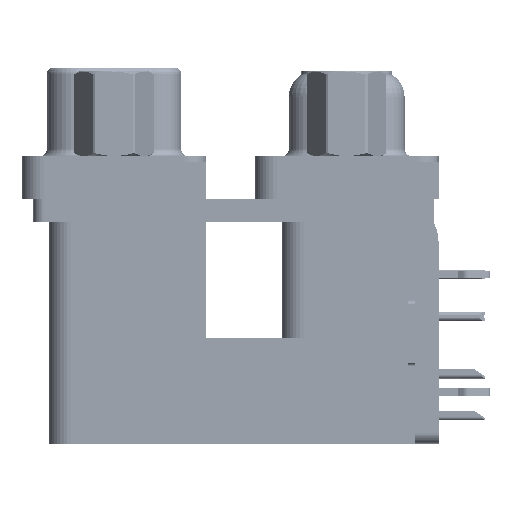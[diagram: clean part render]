
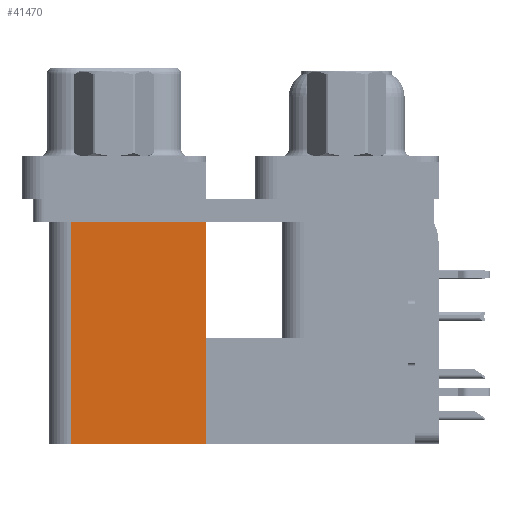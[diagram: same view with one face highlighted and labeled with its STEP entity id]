
A CAD part, left-side view. The second image highlights one B-rep face of the part: STEP entity #41470.
In plain terms, the highlighted planar face has unit normal (-1, 0, 0).
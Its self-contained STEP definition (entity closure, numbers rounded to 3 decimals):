
#2677 = EDGE_CURVE ( 'NONE', #49202, #59503, #44409, .T. ) ;
#3089 = EDGE_CURVE ( 'NONE', #24896, #7739, #49292, .T. ) ;
#5313 = CARTESIAN_POINT ( 'NONE',  ( 3.7, 9.6, -2.5 ) ) ;
#6377 = DIRECTION ( 'NONE',  ( 0., 0., -1. ) ) ;
#7739 = VERTEX_POINT ( 'NONE', #27088 ) ;
#9005 = LINE ( 'NONE', #17838, #18679 ) ;
#10030 = EDGE_LOOP ( 'NONE', ( #37730, #56517, #49188, #27973 ) ) ;
#17838 = CARTESIAN_POINT ( 'NONE',  ( 3.7, 18.8, -19.2 ) ) ;
#18679 = VECTOR ( 'NONE', #46543, 1000. ) ;
#20247 = VECTOR ( 'NONE', #49609, 1000. ) ;
#21953 = CARTESIAN_POINT ( 'NONE',  ( 3.7, 9.6, -19.2 ) ) ;
#22040 = EDGE_CURVE ( 'NONE', #24896, #49202, #60112, .T. ) ;
#24652 = DIRECTION ( 'NONE',  ( 1., 0., 0. ) ) ;
#24896 = VERTEX_POINT ( 'NONE', #49937 ) ;
#27088 = CARTESIAN_POINT ( 'NONE',  ( 3.7, 18.8, -19.2 ) ) ;
#27973 = ORIENTED_EDGE ( 'NONE', *, *, #22040, .T. ) ;
#29318 = VECTOR ( 'NONE', #58591, 1000. ) ;
#30328 = PLANE ( 'NONE',  #56563 ) ;
#34440 = CARTESIAN_POINT ( 'NONE',  ( 3.7, 9.6, -19.2 ) ) ;
#35237 = DIRECTION ( 'NONE',  ( 0., 0., 1. ) ) ;
#37730 = ORIENTED_EDGE ( 'NONE', *, *, #2677, .T. ) ;
#38552 = FACE_OUTER_BOUND ( 'NONE', #10030, .T. ) ;
#41470 = ADVANCED_FACE ( 'NONE', ( #38552 ), #30328, .F. ) ;
#44409 = LINE ( 'NONE', #5313, #29318 ) ;
#46207 = CARTESIAN_POINT ( 'NONE',  ( 3.7, 9.6, -2.5 ) ) ;
#46543 = DIRECTION ( 'NONE',  ( 0., 0., 1. ) ) ;
#47544 = VECTOR ( 'NONE', #35237, 1000. ) ;
#48979 = CARTESIAN_POINT ( 'NONE',  ( 3.7, 9.6, -19.2 ) ) ;
#49188 = ORIENTED_EDGE ( 'NONE', *, *, #3089, .F. ) ;
#49202 = VERTEX_POINT ( 'NONE', #46207 ) ;
#49292 = LINE ( 'NONE', #48979, #20247 ) ;
#49609 = DIRECTION ( 'NONE',  ( 0., 1., 0. ) ) ;
#49937 = CARTESIAN_POINT ( 'NONE',  ( 3.7, 9.6, -19.2 ) ) ;
#52349 = EDGE_CURVE ( 'NONE', #7739, #59503, #9005, .T. ) ;
#56517 = ORIENTED_EDGE ( 'NONE', *, *, #52349, .F. ) ;
#56563 = AXIS2_PLACEMENT_3D ( 'NONE', #34440, #24652, #6377 ) ;
#57976 = CARTESIAN_POINT ( 'NONE',  ( 3.7, 18.8, -2.5 ) ) ;
#58591 = DIRECTION ( 'NONE',  ( 0., 1., 0. ) ) ;
#59503 = VERTEX_POINT ( 'NONE', #57976 ) ;
#60112 = LINE ( 'NONE', #21953, #47544 ) ;
